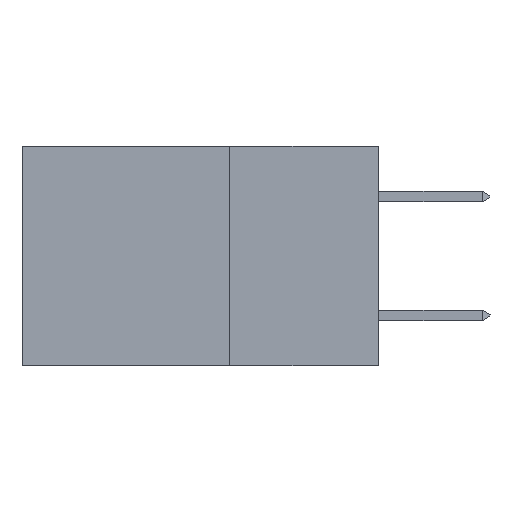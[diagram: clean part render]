
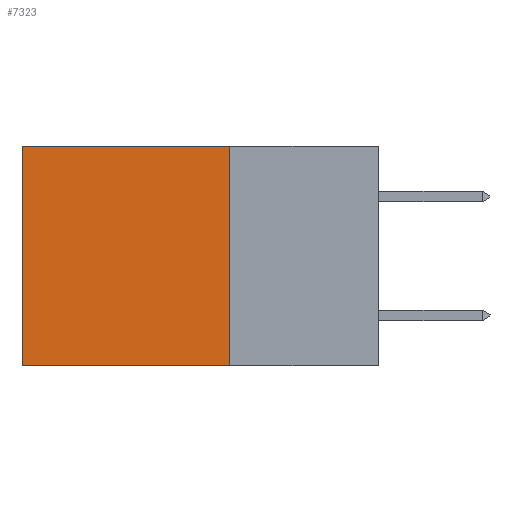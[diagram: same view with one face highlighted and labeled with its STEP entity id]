
A CAD part, left-side view. The second image highlights one B-rep face of the part: STEP entity #7323.
In plain terms, the highlighted planar face has unit normal (-1, 0, 0).
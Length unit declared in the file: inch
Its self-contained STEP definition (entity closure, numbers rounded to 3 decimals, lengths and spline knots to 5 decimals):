
#2275 = VERTEX_POINT ( 'NONE', #9990 ) ;
#3406 = DIRECTION ( 'NONE',  ( 0., 0., -1. ) ) ;
#3517 = EDGE_CURVE ( 'NONE', #2275, #18439, #16835, .T. ) ;
#5071 = DIRECTION ( 'NONE',  ( 0., 1., 0. ) ) ;
#5114 = FACE_OUTER_BOUND ( 'NONE', #18975, .T. ) ;
#5637 = EDGE_CURVE ( 'NONE', #15122, #12138, #18786, .T. ) ;
#5981 = VECTOR ( 'NONE', #3406, 39.37008 ) ;
#6783 = EDGE_CURVE ( 'NONE', #18439, #12138, #20229, .T. ) ;
#7008 = CARTESIAN_POINT ( 'NONE',  ( 0.298, 0.25, 0. ) ) ;
#7323 = ADVANCED_FACE ( 'NONE', ( #5114 ), #12742, .F. ) ;
#7533 = ORIENTED_EDGE ( 'NONE', *, *, #3517, .F. ) ;
#8237 = DIRECTION ( 'NONE',  ( 0., 0., -1. ) ) ;
#9511 = ORIENTED_EDGE ( 'NONE', *, *, #5637, .T. ) ;
#9990 = CARTESIAN_POINT ( 'NONE',  ( 0.298, 0.25, 0. ) ) ;
#10583 = CARTESIAN_POINT ( 'NONE',  ( 0.298, 0.25, 0. ) ) ;
#12054 = ORIENTED_EDGE ( 'NONE', *, *, #20370, .T. ) ;
#12138 = VERTEX_POINT ( 'NONE', #13392 ) ;
#12455 = VECTOR ( 'NONE', #5071, 39.37008 ) ;
#12742 = PLANE ( 'NONE',  #19506 ) ;
#13392 = CARTESIAN_POINT ( 'NONE',  ( 0.298, 0.6, -0.37 ) ) ;
#15122 = VERTEX_POINT ( 'NONE', #19282 ) ;
#15414 = VECTOR ( 'NONE', #15484, 39.37008 ) ;
#15484 = DIRECTION ( 'NONE',  ( 0., 1., 0. ) ) ;
#16624 = DIRECTION ( 'NONE',  ( 1., 0., 0. ) ) ;
#16835 = LINE ( 'NONE', #22385, #5981 ) ;
#18439 = VERTEX_POINT ( 'NONE', #24869 ) ;
#18500 = VECTOR ( 'NONE', #8237, 39.37008 ) ;
#18786 = LINE ( 'NONE', #19552, #18500 ) ;
#18975 = EDGE_LOOP ( 'NONE', ( #9511, #19021, #7533, #12054 ) ) ;
#19021 = ORIENTED_EDGE ( 'NONE', *, *, #6783, .F. ) ;
#19282 = CARTESIAN_POINT ( 'NONE',  ( 0.298, 0.6, 0. ) ) ;
#19447 = CARTESIAN_POINT ( 'NONE',  ( 0.298, 0.25, -0.37 ) ) ;
#19506 = AXIS2_PLACEMENT_3D ( 'NONE', #7008, #16624, #20427 ) ;
#19552 = CARTESIAN_POINT ( 'NONE',  ( 0.298, 0.6, 0. ) ) ;
#20229 = LINE ( 'NONE', #19447, #15414 ) ;
#20370 = EDGE_CURVE ( 'NONE', #2275, #15122, #22407, .T. ) ;
#20427 = DIRECTION ( 'NONE',  ( 0., 0., -1. ) ) ;
#22385 = CARTESIAN_POINT ( 'NONE',  ( 0.298, 0.25, 0. ) ) ;
#22407 = LINE ( 'NONE', #10583, #12455 ) ;
#24869 = CARTESIAN_POINT ( 'NONE',  ( 0.298, 0.25, -0.37 ) ) ;
